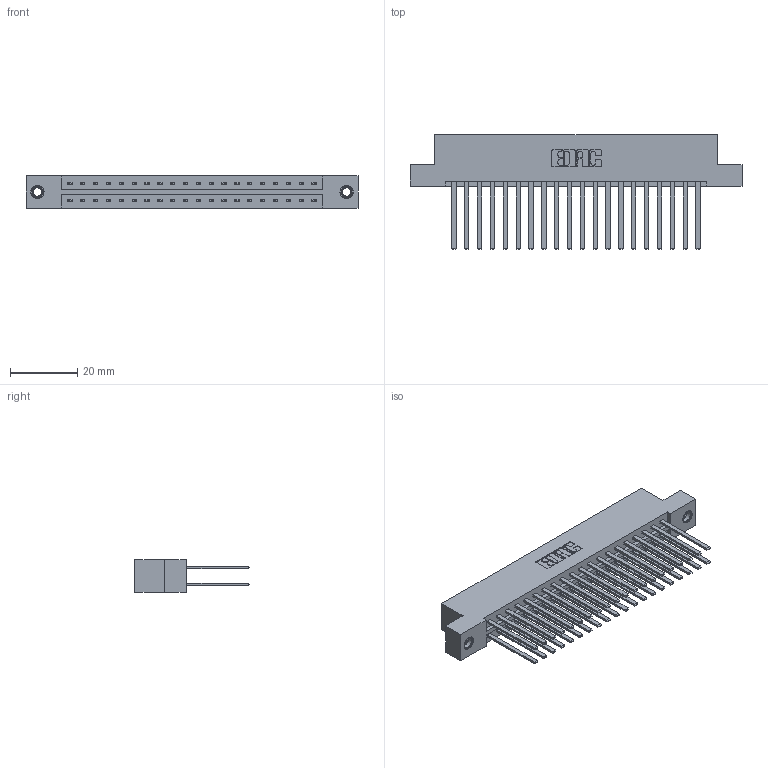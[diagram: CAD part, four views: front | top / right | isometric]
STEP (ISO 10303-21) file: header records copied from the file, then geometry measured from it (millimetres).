
FILE_DESCRIPTION (( 'STEP AP203' ), '1' );
FILE_NAME ('379-040-544-207.STEP', '2020-02-26T17:10:32', ( '' ), ( '' ), 'SwSTEP 2.0', 'SolidWorks 2016', '' );
FILE_SCHEMA (( 'CONFIG_CONTROL_DESIGN' ));
Length unit declared in the file: inch
Products named in the file (4): 379-040-544-207; 379 Part_Flush - .156 Dia - TI; 345-250-001_345-250-005-103; 345-292-001_345-293-144
Assembly tree (43 placements, depth 2):
  379-040-544-207
    379 Part_Flush - .156 Dia - TI
    345-292-001_345-293-144  x40
    345-250-001_345-250-005-103  x2
Bounding box: 98.42 x 33.96 x 9.53 mm (x, y, z)
Volume: 10757.1 mm3; surface area: 13751.7 mm2
Topology: 43 solids, 43 shells, 2014 faces, 5927 edges, 3890 vertices
Faces by surface type: plane 1382, cylinder 616, cone 12, torus 4
Entity records: 16714 total; most frequent: CARTESIAN_POINT 2777, ORIENTED_EDGE 2706, DIRECTION 2439, EDGE_CURVE 1353, LINE 1209, VECTOR 1209, VERTEX_POINT 896, AXIS2_PLACEMENT_3D 615
